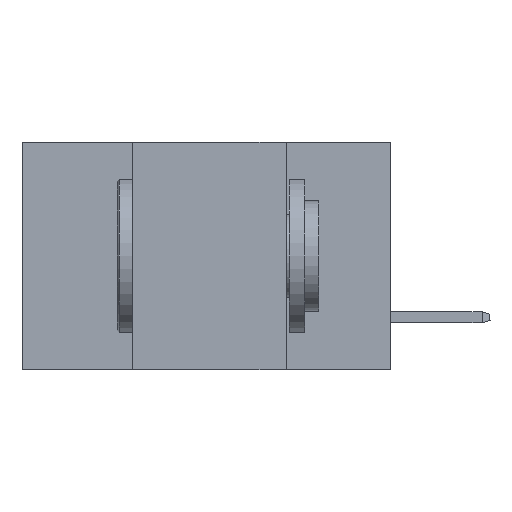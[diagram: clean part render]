
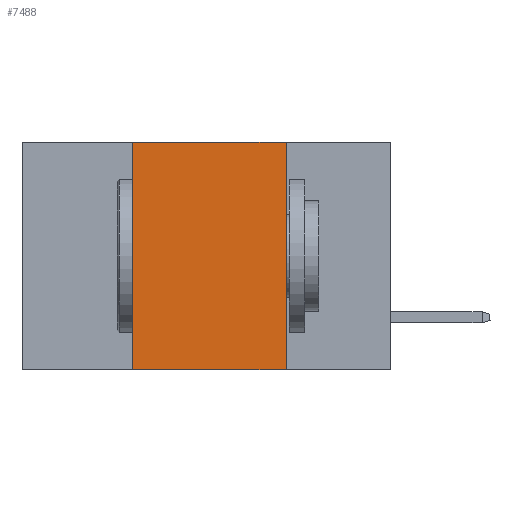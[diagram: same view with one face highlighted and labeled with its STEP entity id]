
A CAD part, left-side view. The second image highlights one B-rep face of the part: STEP entity #7488.
In plain terms, the highlighted planar face has unit normal (-1, 0, 0).
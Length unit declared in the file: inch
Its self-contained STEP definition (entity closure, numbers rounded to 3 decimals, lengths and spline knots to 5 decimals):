
#183 = VECTOR ( 'NONE', #3669, 39.37008 ) ;
#1015 = LINE ( 'NONE', #7524, #183 ) ;
#1108 = CARTESIAN_POINT ( 'NONE',  ( 0., 0.17, -0.37 ) ) ;
#1529 = VECTOR ( 'NONE', #7225, 39.37008 ) ;
#1563 = AXIS2_PLACEMENT_3D ( 'NONE', #12850, #8935, #2407 ) ;
#1654 = EDGE_CURVE ( 'NONE', #2548, #10871, #10768, .T. ) ;
#2336 = FACE_OUTER_BOUND ( 'NONE', #9673, .T. ) ;
#2407 = DIRECTION ( 'NONE',  ( 0., 0., -1. ) ) ;
#2548 = VERTEX_POINT ( 'NONE', #5201 ) ;
#3669 = DIRECTION ( 'NONE',  ( 0., -1., 0. ) ) ;
#3994 = DIRECTION ( 'NONE',  ( 0., -1., 0. ) ) ;
#5201 = CARTESIAN_POINT ( 'NONE',  ( 0., 0.42, -0.37 ) ) ;
#5423 = ORIENTED_EDGE ( 'NONE', *, *, #6360, .F. ) ;
#5787 = VERTEX_POINT ( 'NONE', #1108 ) ;
#6015 = LINE ( 'NONE', #13513, #8695 ) ;
#6274 = PLANE ( 'NONE',  #1563 ) ;
#6360 = EDGE_CURVE ( 'NONE', #7809, #5787, #6461, .T. ) ;
#6461 = LINE ( 'NONE', #14087, #12857 ) ;
#7225 = DIRECTION ( 'NONE',  ( 0., 0., 1. ) ) ;
#7368 = EDGE_CURVE ( 'NONE', #2548, #5787, #6015, .T. ) ;
#7488 = ADVANCED_FACE ( 'NONE', ( #2336 ), #6274, .F. ) ;
#7524 = CARTESIAN_POINT ( 'NONE',  ( 0., 0.6, 0. ) ) ;
#7809 = VERTEX_POINT ( 'NONE', #9087 ) ;
#8695 = VECTOR ( 'NONE', #3994, 39.37008 ) ;
#8935 = DIRECTION ( 'NONE',  ( 1., 0., 0. ) ) ;
#9087 = CARTESIAN_POINT ( 'NONE',  ( 0., 0.17, 0. ) ) ;
#9673 = EDGE_LOOP ( 'NONE', ( #5423, #11011, #9732, #14466 ) ) ;
#9679 = EDGE_CURVE ( 'NONE', #10871, #7809, #1015, .T. ) ;
#9732 = ORIENTED_EDGE ( 'NONE', *, *, #1654, .F. ) ;
#10768 = LINE ( 'NONE', #12485, #1529 ) ;
#10871 = VERTEX_POINT ( 'NONE', #11358 ) ;
#11011 = ORIENTED_EDGE ( 'NONE', *, *, #9679, .F. ) ;
#11358 = CARTESIAN_POINT ( 'NONE',  ( 0., 0.42, 0. ) ) ;
#12485 = CARTESIAN_POINT ( 'NONE',  ( 0., 0.42, 0. ) ) ;
#12816 = DIRECTION ( 'NONE',  ( 0., 0., -1. ) ) ;
#12850 = CARTESIAN_POINT ( 'NONE',  ( 0., 0.6, 0. ) ) ;
#12857 = VECTOR ( 'NONE', #12816, 39.37008 ) ;
#13513 = CARTESIAN_POINT ( 'NONE',  ( 0., 0.6, -0.37 ) ) ;
#14087 = CARTESIAN_POINT ( 'NONE',  ( 0., 0.17, 0. ) ) ;
#14466 = ORIENTED_EDGE ( 'NONE', *, *, #7368, .T. ) ;
